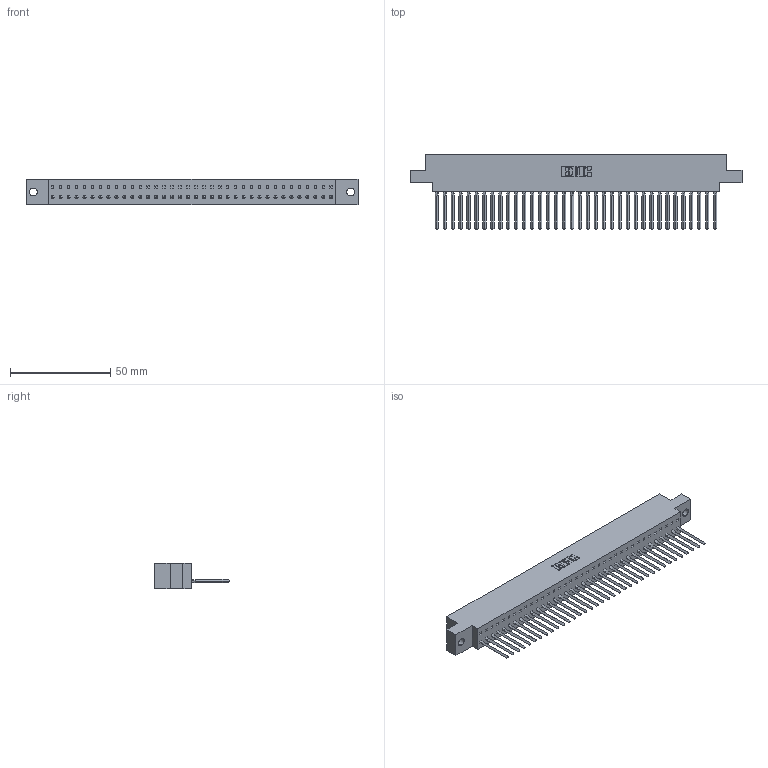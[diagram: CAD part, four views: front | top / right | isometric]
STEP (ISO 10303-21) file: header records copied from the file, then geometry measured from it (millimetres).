
FILE_DESCRIPTION (( 'STEP AP203' ), '1' );
FILE_NAME ('317-036-541-604.STEP', '2020-02-27T22:38:31', ( '' ), ( '' ), 'SwSTEP 2.0', 'SolidWorks 2016', '' );
FILE_SCHEMA (( 'CONFIG_CONTROL_DESIGN' ));
Length unit declared in the file: inch
Products named in the file (3): 317-036-541-604; 317 Part_.156 Dia - TH; 317-290-002_541
Assembly tree (37 placements, depth 2):
  317-036-541-604
    317 Part_.156 Dia - TH
    317-290-002_541  x36
Bounding box: 165.35 x 37.34 x 12.7 mm (x, y, z)
Volume: 26542.5 mm3; surface area: 37124.3 mm2
Topology: 37 solids, 37 shells, 5574 faces, 15899 edges, 10334 vertices
Faces by surface type: plane 4522, cylinder 908, bspline 144
Entity records: 53274 total; most frequent: CARTESIAN_POINT 10109, ORIENTED_EDGE 9398, DIRECTION 7715, EDGE_CURVE 4699, VECTOR 4335, LINE 4335, VERTEX_POINT 3124, AXIS2_PLACEMENT_3D 1690
